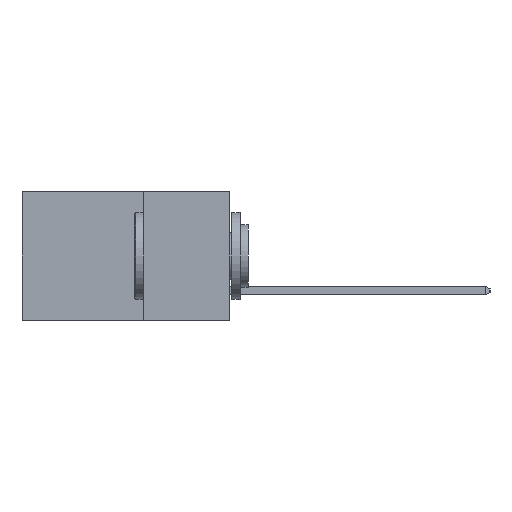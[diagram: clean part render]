
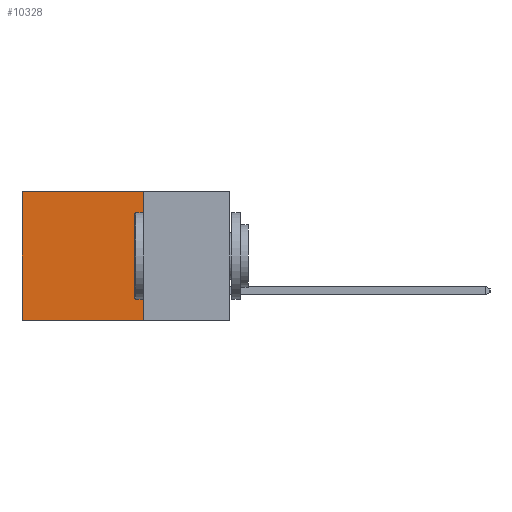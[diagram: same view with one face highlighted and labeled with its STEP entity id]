
A CAD part, left-side view. The second image highlights one B-rep face of the part: STEP entity #10328.
In plain terms, the highlighted planar face has unit normal (-1, 0, 0).
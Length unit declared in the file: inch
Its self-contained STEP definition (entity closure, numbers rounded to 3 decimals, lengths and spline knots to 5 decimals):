
#833 = LINE ( 'NONE', #1924, #8517 ) ;
#909 = DIRECTION ( 'NONE',  ( 0., 0., -1. ) ) ;
#1528 = CARTESIAN_POINT ( 'NONE',  ( 0.298, 0.25, 0. ) ) ;
#1924 = CARTESIAN_POINT ( 'NONE',  ( 0.298, 0.25, -0.37 ) ) ;
#2424 = ORIENTED_EDGE ( 'NONE', *, *, #5651, .T. ) ;
#2573 = LINE ( 'NONE', #8623, #4304 ) ;
#2639 = CARTESIAN_POINT ( 'NONE',  ( 0.298, 0.6, 0. ) ) ;
#3472 = ORIENTED_EDGE ( 'NONE', *, *, #4089, .T. ) ;
#3538 = AXIS2_PLACEMENT_3D ( 'NONE', #10068, #5182, #12025 ) ;
#3660 = ORIENTED_EDGE ( 'NONE', *, *, #7184, .F. ) ;
#3800 = VECTOR ( 'NONE', #11307, 39.37008 ) ;
#3964 = DIRECTION ( 'NONE',  ( 0., 1., 0. ) ) ;
#4080 = LINE ( 'NONE', #1528, #11612 ) ;
#4089 = EDGE_CURVE ( 'NONE', #9973, #10019, #2573, .T. ) ;
#4304 = VECTOR ( 'NONE', #10777, 39.37008 ) ;
#4373 = ORIENTED_EDGE ( 'NONE', *, *, #12687, .F. ) ;
#4658 = VERTEX_POINT ( 'NONE', #9059 ) ;
#4946 = FACE_OUTER_BOUND ( 'NONE', #6769, .T. ) ;
#5182 = DIRECTION ( 'NONE',  ( 1., 0., 0. ) ) ;
#5651 = EDGE_CURVE ( 'NONE', #9787, #9973, #9652, .T. ) ;
#6769 = EDGE_LOOP ( 'NONE', ( #3472, #4373, #3660, #2424 ) ) ;
#7184 = EDGE_CURVE ( 'NONE', #9787, #4658, #4080, .T. ) ;
#8517 = VECTOR ( 'NONE', #3964, 39.37008 ) ;
#8623 = CARTESIAN_POINT ( 'NONE',  ( 0.298, 0.6, 0. ) ) ;
#9059 = CARTESIAN_POINT ( 'NONE',  ( 0.298, 0.25, -0.37 ) ) ;
#9652 = LINE ( 'NONE', #11047, #3800 ) ;
#9787 = VERTEX_POINT ( 'NONE', #12209 ) ;
#9973 = VERTEX_POINT ( 'NONE', #2639 ) ;
#10019 = VERTEX_POINT ( 'NONE', #10558 ) ;
#10068 = CARTESIAN_POINT ( 'NONE',  ( 0.298, 0.25, 0. ) ) ;
#10328 = ADVANCED_FACE ( 'NONE', ( #4946 ), #11048, .F. ) ;
#10558 = CARTESIAN_POINT ( 'NONE',  ( 0.298, 0.6, -0.37 ) ) ;
#10777 = DIRECTION ( 'NONE',  ( 0., 0., -1. ) ) ;
#11047 = CARTESIAN_POINT ( 'NONE',  ( 0.298, 0.25, 0. ) ) ;
#11048 = PLANE ( 'NONE',  #3538 ) ;
#11307 = DIRECTION ( 'NONE',  ( 0., 1., 0. ) ) ;
#11612 = VECTOR ( 'NONE', #909, 39.37008 ) ;
#12025 = DIRECTION ( 'NONE',  ( 0., 0., -1. ) ) ;
#12209 = CARTESIAN_POINT ( 'NONE',  ( 0.298, 0.25, 0. ) ) ;
#12687 = EDGE_CURVE ( 'NONE', #4658, #10019, #833, .T. ) ;
